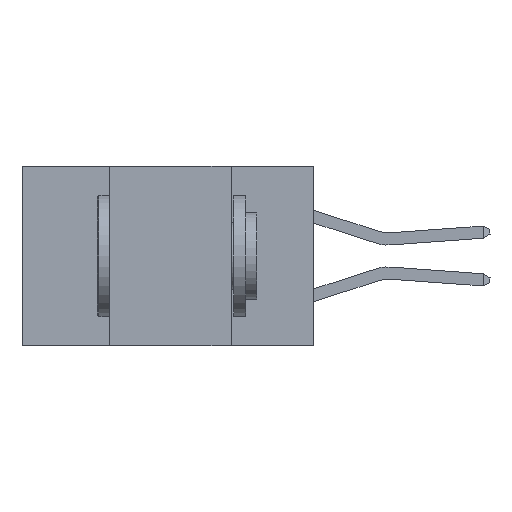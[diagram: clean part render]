
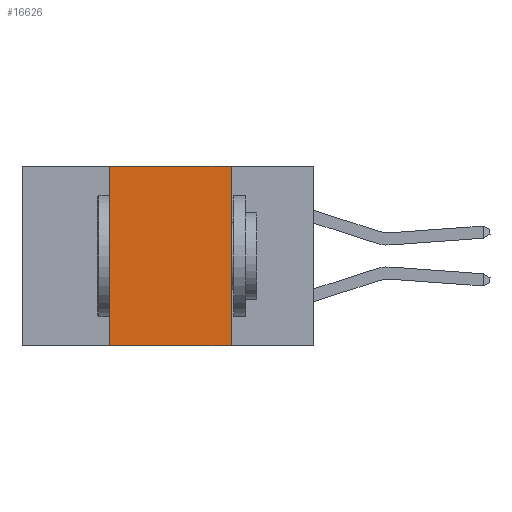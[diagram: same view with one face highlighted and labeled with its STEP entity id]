
A CAD part, left-side view. The second image highlights one B-rep face of the part: STEP entity #16626.
In plain terms, the highlighted planar face has unit normal (-1, 0, 0).
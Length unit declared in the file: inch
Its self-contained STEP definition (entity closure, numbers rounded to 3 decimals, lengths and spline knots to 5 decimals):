
#2363 = CARTESIAN_POINT ( 'NONE',  ( 0., 0.42, 0. ) ) ;
#3277 = DIRECTION ( 'NONE',  ( 0., -1., 0. ) ) ;
#3652 = LINE ( 'NONE', #3915, #22386 ) ;
#3915 = CARTESIAN_POINT ( 'NONE',  ( 0., 0.17, 0. ) ) ;
#3948 = CARTESIAN_POINT ( 'NONE',  ( 0., 0.42, 0. ) ) ;
#4014 = VERTEX_POINT ( 'NONE', #14035 ) ;
#4087 = VECTOR ( 'NONE', #3277, 39.37008 ) ;
#5524 = CARTESIAN_POINT ( 'NONE',  ( 0., 0.6, 0. ) ) ;
#5570 = DIRECTION ( 'NONE',  ( 0., 0., -1. ) ) ;
#6076 = CARTESIAN_POINT ( 'NONE',  ( 0., 0.17, 0. ) ) ;
#6787 = LINE ( 'NONE', #3948, #15894 ) ;
#7095 = EDGE_CURVE ( 'NONE', #18217, #23097, #10130, .T. ) ;
#9554 = VECTOR ( 'NONE', #18327, 39.37008 ) ;
#10028 = DIRECTION ( 'NONE',  ( 0., 0., -1. ) ) ;
#10130 = LINE ( 'NONE', #5524, #9554 ) ;
#10789 = EDGE_CURVE ( 'NONE', #4014, #21947, #14038, .T. ) ;
#11764 = DIRECTION ( 'NONE',  ( 1., 0., 0. ) ) ;
#11968 = EDGE_LOOP ( 'NONE', ( #22773, #11989, #15266, #15527 ) ) ;
#11989 = ORIENTED_EDGE ( 'NONE', *, *, #7095, .F. ) ;
#14035 = CARTESIAN_POINT ( 'NONE',  ( 0., 0.42, -0.37 ) ) ;
#14038 = LINE ( 'NONE', #14222, #4087 ) ;
#14222 = CARTESIAN_POINT ( 'NONE',  ( 0., 0.6, -0.37 ) ) ;
#15266 = ORIENTED_EDGE ( 'NONE', *, *, #17405, .F. ) ;
#15357 = CARTESIAN_POINT ( 'NONE',  ( 0., 0.6, 0. ) ) ;
#15527 = ORIENTED_EDGE ( 'NONE', *, *, #10789, .T. ) ;
#15894 = VECTOR ( 'NONE', #16675, 39.37008 ) ;
#16626 = ADVANCED_FACE ( 'NONE', ( #21278 ), #20338, .F. ) ;
#16675 = DIRECTION ( 'NONE',  ( 0., 0., 1. ) ) ;
#17405 = EDGE_CURVE ( 'NONE', #4014, #18217, #6787, .T. ) ;
#17782 = EDGE_CURVE ( 'NONE', #23097, #21947, #3652, .T. ) ;
#18217 = VERTEX_POINT ( 'NONE', #2363 ) ;
#18327 = DIRECTION ( 'NONE',  ( 0., -1., 0. ) ) ;
#19259 = CARTESIAN_POINT ( 'NONE',  ( 0., 0.17, -0.37 ) ) ;
#20338 = PLANE ( 'NONE',  #22318 ) ;
#21278 = FACE_OUTER_BOUND ( 'NONE', #11968, .T. ) ;
#21947 = VERTEX_POINT ( 'NONE', #19259 ) ;
#22318 = AXIS2_PLACEMENT_3D ( 'NONE', #15357, #11764, #10028 ) ;
#22386 = VECTOR ( 'NONE', #5570, 39.37008 ) ;
#22773 = ORIENTED_EDGE ( 'NONE', *, *, #17782, .F. ) ;
#23097 = VERTEX_POINT ( 'NONE', #6076 ) ;
